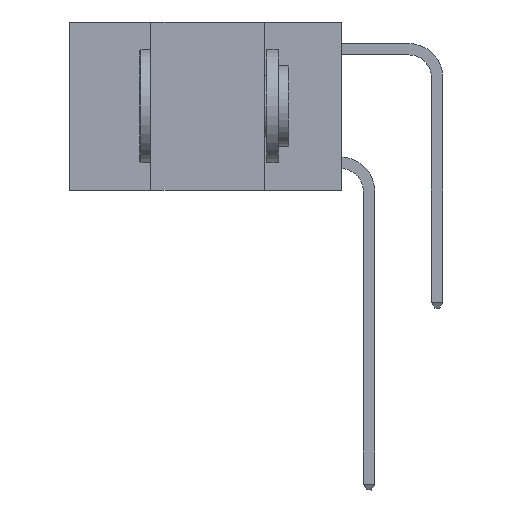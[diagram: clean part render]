
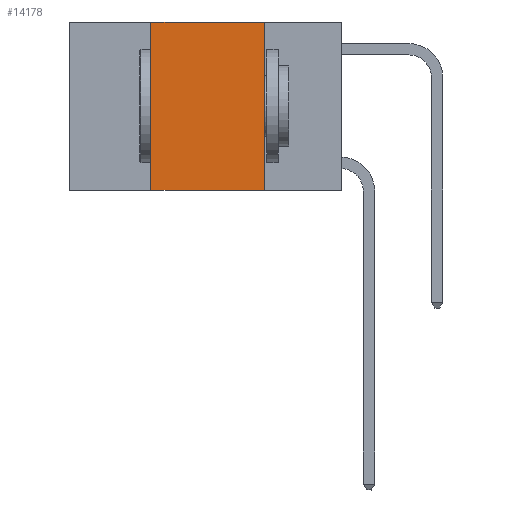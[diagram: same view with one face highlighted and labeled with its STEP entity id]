
A CAD part, left-side view. The second image highlights one B-rep face of the part: STEP entity #14178.
In plain terms, the highlighted planar face has unit normal (-1, 0, 0).
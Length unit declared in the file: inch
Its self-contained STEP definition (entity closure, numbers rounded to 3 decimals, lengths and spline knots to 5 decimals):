
#1675 = CARTESIAN_POINT ( 'NONE',  ( 0., 0.17, -0.37 ) ) ;
#4676 = ORIENTED_EDGE ( 'NONE', *, *, #8775, .F. ) ;
#5894 = CARTESIAN_POINT ( 'NONE',  ( 0., 0.6, 0. ) ) ;
#5980 = VECTOR ( 'NONE', #24499, 39.37008 ) ;
#6637 = FACE_OUTER_BOUND ( 'NONE', #17376, .T. ) ;
#6800 = DIRECTION ( 'NONE',  ( 0., 0., 1. ) ) ;
#7716 = LINE ( 'NONE', #25943, #21653 ) ;
#8243 = PLANE ( 'NONE',  #20212 ) ;
#8775 = EDGE_CURVE ( 'NONE', #19400, #17921, #10970, .T. ) ;
#9391 = CARTESIAN_POINT ( 'NONE',  ( 0., 0.6, 0. ) ) ;
#10970 = LINE ( 'NONE', #20786, #11758 ) ;
#11758 = VECTOR ( 'NONE', #6800, 39.37008 ) ;
#12330 = EDGE_CURVE ( 'NONE', #17921, #14636, #22619, .T. ) ;
#12872 = ORIENTED_EDGE ( 'NONE', *, *, #12330, .F. ) ;
#13345 = DIRECTION ( 'NONE',  ( 1., 0., 0. ) ) ;
#14178 = ADVANCED_FACE ( 'NONE', ( #6637 ), #8243, .F. ) ;
#14636 = VERTEX_POINT ( 'NONE', #30063 ) ;
#16437 = ORIENTED_EDGE ( 'NONE', *, *, #16722, .F. ) ;
#16722 = EDGE_CURVE ( 'NONE', #14636, #27614, #24296, .T. ) ;
#17376 = EDGE_LOOP ( 'NONE', ( #16437, #12872, #4676, #26996 ) ) ;
#17921 = VERTEX_POINT ( 'NONE', #31586 ) ;
#18008 = EDGE_CURVE ( 'NONE', #19400, #27614, #7716, .T. ) ;
#19400 = VERTEX_POINT ( 'NONE', #23195 ) ;
#20212 = AXIS2_PLACEMENT_3D ( 'NONE', #5894, #13345, #30756 ) ;
#20786 = CARTESIAN_POINT ( 'NONE',  ( 0., 0.42, 0. ) ) ;
#21653 = VECTOR ( 'NONE', #24077, 39.37008 ) ;
#22619 = LINE ( 'NONE', #9391, #5980 ) ;
#23195 = CARTESIAN_POINT ( 'NONE',  ( 0., 0.42, -0.37 ) ) ;
#23916 = VECTOR ( 'NONE', #30693, 39.37008 ) ;
#24077 = DIRECTION ( 'NONE',  ( 0., -1., 0. ) ) ;
#24296 = LINE ( 'NONE', #26108, #23916 ) ;
#24499 = DIRECTION ( 'NONE',  ( 0., -1., 0. ) ) ;
#25943 = CARTESIAN_POINT ( 'NONE',  ( 0., 0.6, -0.37 ) ) ;
#26108 = CARTESIAN_POINT ( 'NONE',  ( 0., 0.17, 0. ) ) ;
#26996 = ORIENTED_EDGE ( 'NONE', *, *, #18008, .T. ) ;
#27614 = VERTEX_POINT ( 'NONE', #1675 ) ;
#30063 = CARTESIAN_POINT ( 'NONE',  ( 0., 0.17, 0. ) ) ;
#30693 = DIRECTION ( 'NONE',  ( 0., 0., -1. ) ) ;
#30756 = DIRECTION ( 'NONE',  ( 0., 0., -1. ) ) ;
#31586 = CARTESIAN_POINT ( 'NONE',  ( 0., 0.42, 0. ) ) ;
